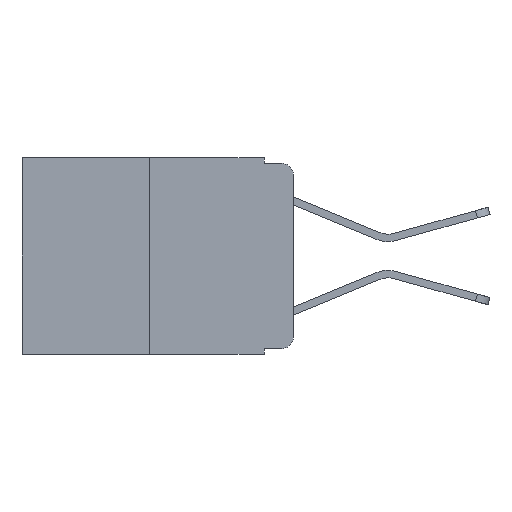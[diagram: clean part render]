
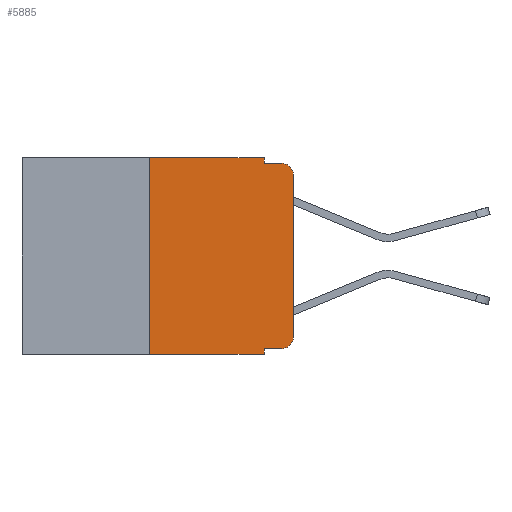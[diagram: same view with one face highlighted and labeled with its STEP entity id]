
A CAD part, left-side view. The second image highlights one B-rep face of the part: STEP entity #5885.
In plain terms, the highlighted planar face has unit normal (-1, 0, 0).
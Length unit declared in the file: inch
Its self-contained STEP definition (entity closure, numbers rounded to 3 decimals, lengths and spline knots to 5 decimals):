
#325 = ORIENTED_EDGE ( 'NONE', *, *, #4059, .T. ) ;
#648 = VERTEX_POINT ( 'NONE', #5877 ) ;
#703 = ORIENTED_EDGE ( 'NONE', *, *, #2180, .F. ) ;
#1105 = CARTESIAN_POINT ( 'NONE',  ( 0., 0.051, -0.333 ) ) ;
#1347 = VERTEX_POINT ( 'NONE', #23679 ) ;
#1580 = LINE ( 'NONE', #19076, #16516 ) ;
#1725 = CARTESIAN_POINT ( 'NONE',  ( 0., 0.473, 0. ) ) ;
#2180 = EDGE_CURVE ( 'NONE', #648, #2262, #12534, .T. ) ;
#2262 = VERTEX_POINT ( 'NONE', #20859 ) ;
#2768 = VECTOR ( 'NONE', #9136, 39.37008 ) ;
#3032 = ORIENTED_EDGE ( 'NONE', *, *, #6553, .T. ) ;
#3056 = CARTESIAN_POINT ( 'NONE',  ( 0., 0.051, -0.333 ) ) ;
#3563 = EDGE_CURVE ( 'NONE', #7003, #11128, #1580, .T. ) ;
#3731 = DIRECTION ( 'NONE',  ( 0., 0., -1. ) ) ;
#3781 = DIRECTION ( 'NONE',  ( 1., 0., 0. ) ) ;
#3899 = ORIENTED_EDGE ( 'NONE', *, *, #17003, .F. ) ;
#4059 = EDGE_CURVE ( 'NONE', #12356, #14800, #9626, .T. ) ;
#5147 = CARTESIAN_POINT ( 'NONE',  ( 0., 0.02, -0.03 ) ) ;
#5228 = ORIENTED_EDGE ( 'NONE', *, *, #18081, .T. ) ;
#5837 = ORIENTED_EDGE ( 'NONE', *, *, #3563, .F. ) ;
#5848 = AXIS2_PLACEMENT_3D ( 'NONE', #1725, #3781, #17286 ) ;
#5877 = CARTESIAN_POINT ( 'NONE',  ( 0., 0.051, 0. ) ) ;
#5885 = ADVANCED_FACE ( 'NONE', ( #5945 ), #13420, .F. ) ;
#5910 = DIRECTION ( 'NONE',  ( -1., 0., 0. ) ) ;
#5945 = FACE_OUTER_BOUND ( 'NONE', #15777, .T. ) ;
#6168 = AXIS2_PLACEMENT_3D ( 'NONE', #17426, #5910, #19338 ) ;
#6553 = EDGE_CURVE ( 'NONE', #23496, #12356, #24860, .T. ) ;
#7003 = VERTEX_POINT ( 'NONE', #1105 ) ;
#7089 = DIRECTION ( 'NONE',  ( 0., 0., -1. ) ) ;
#7837 = DIRECTION ( 'NONE',  ( 0., -1., 0. ) ) ;
#8325 = AXIS2_PLACEMENT_3D ( 'NONE', #5147, #18578, #7089 ) ;
#9136 = DIRECTION ( 'NONE',  ( 0., 0., -1. ) ) ;
#9286 = LINE ( 'NONE', #17394, #16428 ) ;
#9296 = DIRECTION ( 'NONE',  ( 0., 0., 1. ) ) ;
#9335 = EDGE_CURVE ( 'NONE', #14800, #19886, #18874, .T. ) ;
#9626 = LINE ( 'NONE', #20759, #20401 ) ;
#9641 = VECTOR ( 'NONE', #15813, 39.37008 ) ;
#9668 = DIRECTION ( 'NONE',  ( 0., -1., 0. ) ) ;
#9988 = EDGE_CURVE ( 'NONE', #7003, #23496, #18879, .T. ) ;
#10223 = CARTESIAN_POINT ( 'NONE',  ( 0., 0., -0.313 ) ) ;
#10947 = VECTOR ( 'NONE', #9668, 39.37008 ) ;
#11128 = VERTEX_POINT ( 'NONE', #17238 ) ;
#11197 = ORIENTED_EDGE ( 'NONE', *, *, #9335, .T. ) ;
#12161 = ORIENTED_EDGE ( 'NONE', *, *, #9988, .T. ) ;
#12356 = VERTEX_POINT ( 'NONE', #10223 ) ;
#12534 = LINE ( 'NONE', #20602, #2768 ) ;
#13420 = PLANE ( 'NONE',  #5848 ) ;
#13773 = VECTOR ( 'NONE', #22421, 39.37008 ) ;
#14221 = ORIENTED_EDGE ( 'NONE', *, *, #15761, .F. ) ;
#14800 = VERTEX_POINT ( 'NONE', #20162 ) ;
#15761 = EDGE_CURVE ( 'NONE', #1347, #648, #19798, .T. ) ;
#15777 = EDGE_LOOP ( 'NONE', ( #325, #11197, #3899, #703, #14221, #25054, #5228, #5837, #12161, #3032 ) ) ;
#15813 = DIRECTION ( 'NONE',  ( 0., -1., 0. ) ) ;
#16263 = CARTESIAN_POINT ( 'NONE',  ( 0., 0.25, 0. ) ) ;
#16428 = VECTOR ( 'NONE', #7837, 39.37008 ) ;
#16516 = VECTOR ( 'NONE', #3731, 39.37008 ) ;
#17003 = EDGE_CURVE ( 'NONE', #2262, #19886, #9286, .T. ) ;
#17185 = CARTESIAN_POINT ( 'NONE',  ( 0., 0.25, -0.343 ) ) ;
#17238 = CARTESIAN_POINT ( 'NONE',  ( 0., 0.051, -0.343 ) ) ;
#17286 = DIRECTION ( 'NONE',  ( 0., 0., -1. ) ) ;
#17394 = CARTESIAN_POINT ( 'NONE',  ( 0., 0.051, -0.01 ) ) ;
#17426 = CARTESIAN_POINT ( 'NONE',  ( 0., 0.02, -0.313 ) ) ;
#17754 = CARTESIAN_POINT ( 'NONE',  ( 0., 0.473, 0. ) ) ;
#18049 = VERTEX_POINT ( 'NONE', #17185 ) ;
#18081 = EDGE_CURVE ( 'NONE', #18049, #11128, #20546, .T. ) ;
#18578 = DIRECTION ( 'NONE',  ( -1., 0., 0. ) ) ;
#18719 = CARTESIAN_POINT ( 'NONE',  ( 0., 0.02, -0.01 ) ) ;
#18874 = CIRCLE ( 'NONE', #8325, 0.02 ) ;
#18879 = LINE ( 'NONE', #3056, #13773 ) ;
#19076 = CARTESIAN_POINT ( 'NONE',  ( 0., 0.051, 0. ) ) ;
#19209 = VECTOR ( 'NONE', #21990, 39.37008 ) ;
#19338 = DIRECTION ( 'NONE',  ( 0., 0., -1. ) ) ;
#19798 = LINE ( 'NONE', #17754, #9641 ) ;
#19841 = CARTESIAN_POINT ( 'NONE',  ( 0., 0.02, -0.333 ) ) ;
#19886 = VERTEX_POINT ( 'NONE', #18719 ) ;
#20162 = CARTESIAN_POINT ( 'NONE',  ( 0., 0., -0.03 ) ) ;
#20393 = EDGE_CURVE ( 'NONE', #18049, #1347, #24356, .T. ) ;
#20401 = VECTOR ( 'NONE', #9296, 39.37008 ) ;
#20546 = LINE ( 'NONE', #21129, #10947 ) ;
#20602 = CARTESIAN_POINT ( 'NONE',  ( 0., 0.051, 0. ) ) ;
#20759 = CARTESIAN_POINT ( 'NONE',  ( 0., 0., 0. ) ) ;
#20859 = CARTESIAN_POINT ( 'NONE',  ( 0., 0.051, -0.01 ) ) ;
#21129 = CARTESIAN_POINT ( 'NONE',  ( 0., 0.473, -0.343 ) ) ;
#21990 = DIRECTION ( 'NONE',  ( 0., 0., 1. ) ) ;
#22421 = DIRECTION ( 'NONE',  ( 0., -1., 0. ) ) ;
#23496 = VERTEX_POINT ( 'NONE', #19841 ) ;
#23679 = CARTESIAN_POINT ( 'NONE',  ( 0., 0.25, 0. ) ) ;
#24356 = LINE ( 'NONE', #16263, #19209 ) ;
#24860 = CIRCLE ( 'NONE', #6168, 0.02 ) ;
#25054 = ORIENTED_EDGE ( 'NONE', *, *, #20393, .F. ) ;
